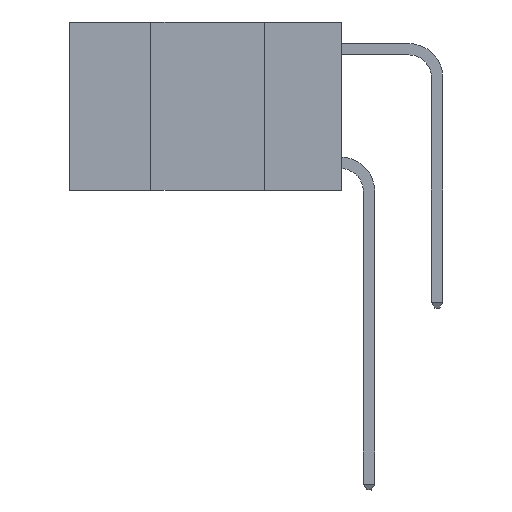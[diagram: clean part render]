
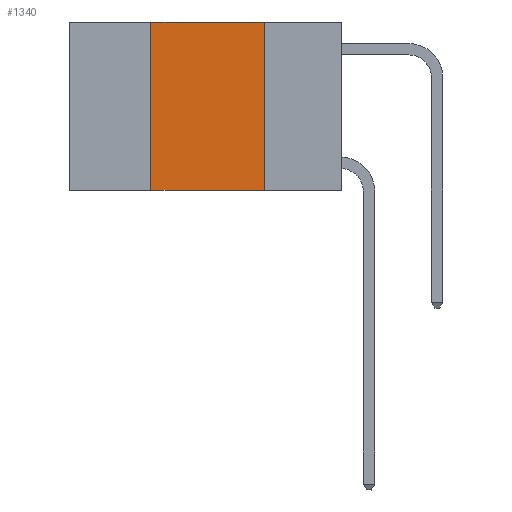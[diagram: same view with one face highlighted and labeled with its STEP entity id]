
A CAD part, left-side view. The second image highlights one B-rep face of the part: STEP entity #1340.
In plain terms, the highlighted planar face has unit normal (-1, 0, 0).
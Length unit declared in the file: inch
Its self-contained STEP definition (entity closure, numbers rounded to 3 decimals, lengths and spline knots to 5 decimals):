
#187 = VERTEX_POINT ( 'NONE', #10437 ) ;
#239 = DIRECTION ( 'NONE',  ( 0., -1., 0. ) ) ;
#588 = VECTOR ( 'NONE', #8127, 39.37008 ) ;
#814 = DIRECTION ( 'NONE',  ( 0., 0., -1. ) ) ;
#885 = FACE_OUTER_BOUND ( 'NONE', #11358, .T. ) ;
#981 = PLANE ( 'NONE',  #7735 ) ;
#1078 = CARTESIAN_POINT ( 'NONE',  ( 0., 0.6, 0. ) ) ;
#1272 = DIRECTION ( 'NONE',  ( 1., 0., 0. ) ) ;
#1340 = ADVANCED_FACE ( 'NONE', ( #885 ), #981, .F. ) ;
#1405 = CARTESIAN_POINT ( 'NONE',  ( 0., 0.42, 0. ) ) ;
#1584 = CARTESIAN_POINT ( 'NONE',  ( 0., 0.6, 0. ) ) ;
#1842 = ORIENTED_EDGE ( 'NONE', *, *, #2525, .F. ) ;
#2157 = ORIENTED_EDGE ( 'NONE', *, *, #5292, .F. ) ;
#2225 = CARTESIAN_POINT ( 'NONE',  ( 0., 0.17, -0.37 ) ) ;
#2525 = EDGE_CURVE ( 'NONE', #5742, #5050, #8975, .T. ) ;
#2766 = EDGE_CURVE ( 'NONE', #5518, #5050, #5761, .T. ) ;
#2835 = CARTESIAN_POINT ( 'NONE',  ( 0., 0.17, 0. ) ) ;
#3287 = VECTOR ( 'NONE', #239, 39.37008 ) ;
#3566 = VECTOR ( 'NONE', #11059, 39.37008 ) ;
#4749 = ORIENTED_EDGE ( 'NONE', *, *, #9665, .F. ) ;
#5050 = VERTEX_POINT ( 'NONE', #2225 ) ;
#5151 = CARTESIAN_POINT ( 'NONE',  ( 0., 0.6, -0.37 ) ) ;
#5292 = EDGE_CURVE ( 'NONE', #187, #5742, #7940, .T. ) ;
#5518 = VERTEX_POINT ( 'NONE', #12248 ) ;
#5742 = VERTEX_POINT ( 'NONE', #11658 ) ;
#5761 = LINE ( 'NONE', #5151, #3287 ) ;
#6490 = VECTOR ( 'NONE', #7511, 39.37008 ) ;
#7209 = ORIENTED_EDGE ( 'NONE', *, *, #2766, .T. ) ;
#7385 = LINE ( 'NONE', #1405, #588 ) ;
#7511 = DIRECTION ( 'NONE',  ( 0., 0., -1. ) ) ;
#7735 = AXIS2_PLACEMENT_3D ( 'NONE', #1078, #1272, #814 ) ;
#7940 = LINE ( 'NONE', #1584, #3566 ) ;
#8127 = DIRECTION ( 'NONE',  ( 0., 0., 1. ) ) ;
#8975 = LINE ( 'NONE', #2835, #6490 ) ;
#9665 = EDGE_CURVE ( 'NONE', #5518, #187, #7385, .T. ) ;
#10437 = CARTESIAN_POINT ( 'NONE',  ( 0., 0.42, 0. ) ) ;
#11059 = DIRECTION ( 'NONE',  ( 0., -1., 0. ) ) ;
#11358 = EDGE_LOOP ( 'NONE', ( #1842, #2157, #4749, #7209 ) ) ;
#11658 = CARTESIAN_POINT ( 'NONE',  ( 0., 0.17, 0. ) ) ;
#12248 = CARTESIAN_POINT ( 'NONE',  ( 0., 0.42, -0.37 ) ) ;
